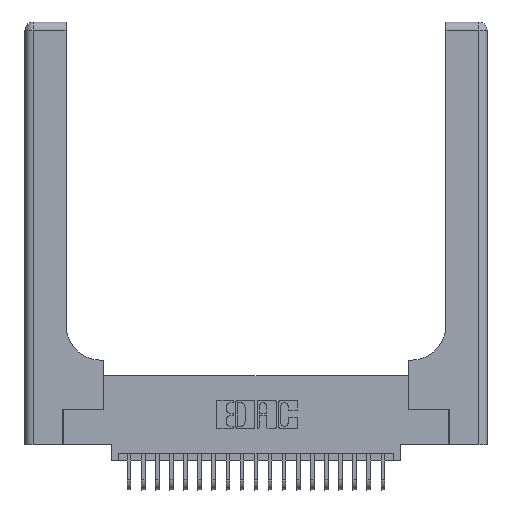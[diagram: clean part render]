
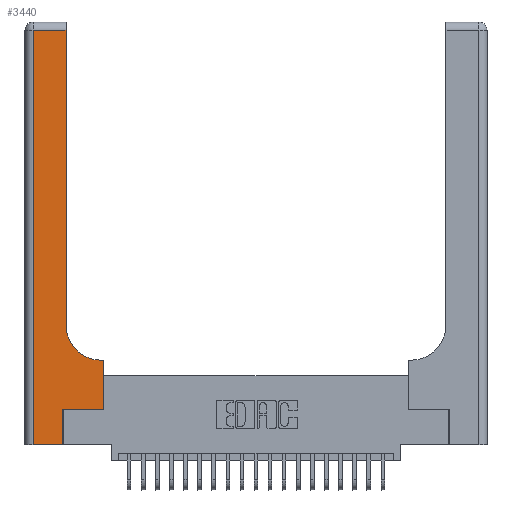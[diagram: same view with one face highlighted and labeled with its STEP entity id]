
A CAD part, top view. The second image highlights one B-rep face of the part: STEP entity #3440.
In plain terms, the highlighted planar face has unit normal (0, 0, 1).
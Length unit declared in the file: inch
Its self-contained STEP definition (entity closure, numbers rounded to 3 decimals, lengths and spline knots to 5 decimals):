
#330 = DIRECTION ( 'NONE',  ( 1., 0., 0. ) ) ;
#437 = EDGE_CURVE ( 'NONE', #22294, #10767, #5562, .T. ) ;
#588 = DIRECTION ( 'NONE',  ( -1., 0., 0. ) ) ;
#1754 = CARTESIAN_POINT ( 'NONE',  ( 0.269, 0., 0.37 ) ) ;
#1964 = LINE ( 'NONE', #12759, #24300 ) ;
#2091 = EDGE_CURVE ( 'NONE', #10767, #2837, #17620, .T. ) ;
#2360 = CARTESIAN_POINT ( 'NONE',  ( 0.5585, 0.25, 0.37 ) ) ;
#2622 = CARTESIAN_POINT ( 'NONE',  ( 0.2915, 3., 0.37 ) ) ;
#2681 = CARTESIAN_POINT ( 'NONE',  ( 0.2915, 0.85, 0.37 ) ) ;
#2837 = VERTEX_POINT ( 'NONE', #22670 ) ;
#3105 = DIRECTION ( 'NONE',  ( 0., -1., 0. ) ) ;
#3440 = ADVANCED_FACE ( 'NONE', ( #18146 ), #17307, .F. ) ;
#3778 = EDGE_CURVE ( 'NONE', #2837, #11213, #22953, .T. ) ;
#3975 = CARTESIAN_POINT ( 'NONE',  ( 0.5415, 0.85, 0.37 ) ) ;
#4216 = ORIENTED_EDGE ( 'NONE', *, *, #14996, .T. ) ;
#4226 = EDGE_CURVE ( 'NONE', #12766, #22267, #15700, .T. ) ;
#4280 = CARTESIAN_POINT ( 'NONE',  ( 0.2915, 0.6, 0.37 ) ) ;
#4638 = VECTOR ( 'NONE', #330, 39.37008 ) ;
#5562 = LINE ( 'NONE', #19575, #4638 ) ;
#6310 = ORIENTED_EDGE ( 'NONE', *, *, #9559, .T. ) ;
#6513 = ORIENTED_EDGE ( 'NONE', *, *, #4226, .T. ) ;
#6647 = ORIENTED_EDGE ( 'NONE', *, *, #8697, .T. ) ;
#7431 = ORIENTED_EDGE ( 'NONE', *, *, #21502, .T. ) ;
#7795 = ORIENTED_EDGE ( 'NONE', *, *, #2091, .T. ) ;
#7855 = DIRECTION ( 'NONE',  ( 0., 0., -1. ) ) ;
#8375 = CARTESIAN_POINT ( 'NONE',  ( 0.5585, 0.6, 0.37 ) ) ;
#8697 = EDGE_CURVE ( 'NONE', #17717, #11500, #18692, .T. ) ;
#9559 = EDGE_CURVE ( 'NONE', #19399, #12766, #19852, .T. ) ;
#9727 = VECTOR ( 'NONE', #23975, 39.37008 ) ;
#9815 = DIRECTION ( 'NONE',  ( 1., 0., 0. ) ) ;
#10159 = VECTOR ( 'NONE', #23957, 39.37008 ) ;
#10358 = CARTESIAN_POINT ( 'NONE',  ( 0.2915, 2.94, 0.37 ) ) ;
#10767 = VERTEX_POINT ( 'NONE', #17962 ) ;
#11213 = VERTEX_POINT ( 'NONE', #2360 ) ;
#11500 = VERTEX_POINT ( 'NONE', #22238 ) ;
#11691 = EDGE_CURVE ( 'NONE', #11500, #22294, #1964, .T. ) ;
#12266 = CARTESIAN_POINT ( 'NONE',  ( 0.5585, 0.25, 0.37 ) ) ;
#12395 = VECTOR ( 'NONE', #13435, 39.37008 ) ;
#12759 = CARTESIAN_POINT ( 'NONE',  ( 0.06, 3., 0.37 ) ) ;
#12766 = VERTEX_POINT ( 'NONE', #14490 ) ;
#13391 = AXIS2_PLACEMENT_3D ( 'NONE', #3975, #7855, #9815 ) ;
#13435 = DIRECTION ( 'NONE',  ( 1., 0., 0. ) ) ;
#13532 = CARTESIAN_POINT ( 'NONE',  ( 0., 3., 0.37 ) ) ;
#13562 = VECTOR ( 'NONE', #588, 39.37008 ) ;
#13612 = DIRECTION ( 'NONE',  ( -1., 0., 0. ) ) ;
#14072 = EDGE_LOOP ( 'NONE', ( #7431, #6647, #19601, #23928, #7795, #18183, #4216, #6310, #6513 ) ) ;
#14113 = CARTESIAN_POINT ( 'NONE',  ( 0.06, 0., 0.37 ) ) ;
#14490 = CARTESIAN_POINT ( 'NONE',  ( 0.5415, 0.6, 0.37 ) ) ;
#14863 = LINE ( 'NONE', #2622, #9727 ) ;
#14996 = EDGE_CURVE ( 'NONE', #11213, #19399, #18034, .T. ) ;
#15700 = CIRCLE ( 'NONE', #13391, 0.25 ) ;
#17307 = PLANE ( 'NONE',  #20479 ) ;
#17620 = LINE ( 'NONE', #1754, #22151 ) ;
#17641 = CARTESIAN_POINT ( 'NONE',  ( 0., 2.94, 0.37 ) ) ;
#17717 = VERTEX_POINT ( 'NONE', #10358 ) ;
#17785 = DIRECTION ( 'NONE',  ( -1., 0., 0. ) ) ;
#17962 = CARTESIAN_POINT ( 'NONE',  ( 0.269, 0., 0.37 ) ) ;
#18034 = LINE ( 'NONE', #12266, #10159 ) ;
#18146 = FACE_OUTER_BOUND ( 'NONE', #14072, .T. ) ;
#18183 = ORIENTED_EDGE ( 'NONE', *, *, #3778, .T. ) ;
#18692 = LINE ( 'NONE', #17641, #13562 ) ;
#18987 = DIRECTION ( 'NONE',  ( 0., 1., 0. ) ) ;
#19255 = DIRECTION ( 'NONE',  ( 0., 0., -1. ) ) ;
#19399 = VERTEX_POINT ( 'NONE', #8375 ) ;
#19575 = CARTESIAN_POINT ( 'NONE',  ( 0., 0., 0.37 ) ) ;
#19601 = ORIENTED_EDGE ( 'NONE', *, *, #11691, .T. ) ;
#19852 = LINE ( 'NONE', #4280, #24047 ) ;
#20479 = AXIS2_PLACEMENT_3D ( 'NONE', #13532, #19255, #13612 ) ;
#21502 = EDGE_CURVE ( 'NONE', #22267, #17717, #14863, .T. ) ;
#22151 = VECTOR ( 'NONE', #18987, 39.37008 ) ;
#22238 = CARTESIAN_POINT ( 'NONE',  ( 0.06, 2.94, 0.37 ) ) ;
#22267 = VERTEX_POINT ( 'NONE', #2681 ) ;
#22294 = VERTEX_POINT ( 'NONE', #14113 ) ;
#22670 = CARTESIAN_POINT ( 'NONE',  ( 0.269, 0.25, 0.37 ) ) ;
#22953 = LINE ( 'NONE', #23029, #12395 ) ;
#23029 = CARTESIAN_POINT ( 'NONE',  ( 0.269, 0.25, 0.37 ) ) ;
#23928 = ORIENTED_EDGE ( 'NONE', *, *, #437, .T. ) ;
#23957 = DIRECTION ( 'NONE',  ( 0., 1., 0. ) ) ;
#23975 = DIRECTION ( 'NONE',  ( 0., 1., 0. ) ) ;
#24047 = VECTOR ( 'NONE', #17785, 39.37008 ) ;
#24300 = VECTOR ( 'NONE', #3105, 39.37008 ) ;
